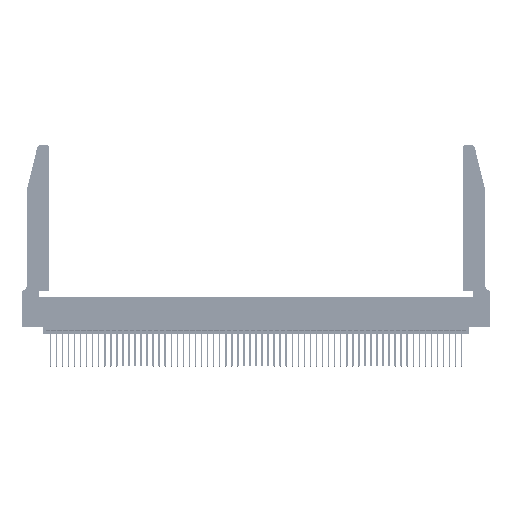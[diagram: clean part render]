
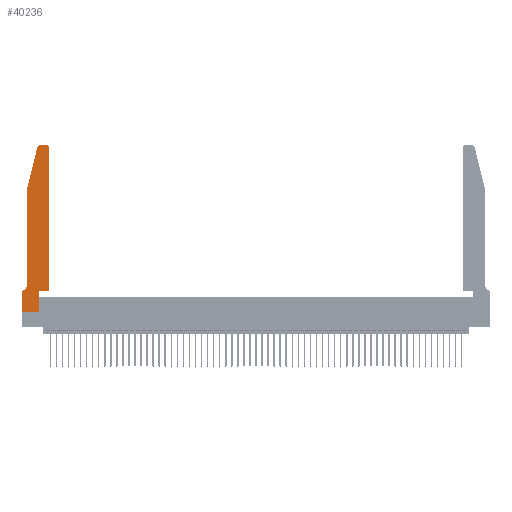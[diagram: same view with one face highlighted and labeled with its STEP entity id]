
A CAD part, top view. The second image highlights one B-rep face of the part: STEP entity #40236.
In plain terms, the highlighted planar face has unit normal (0, 0, 1).
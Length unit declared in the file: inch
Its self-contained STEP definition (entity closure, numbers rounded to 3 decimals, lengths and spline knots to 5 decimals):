
#843 = VERTEX_POINT ( 'NONE', #5994 ) ;
#1290 = VECTOR ( 'NONE', #5709, 39.37008 ) ;
#2330 = CARTESIAN_POINT ( 'NONE',  ( 0.2865, 0.35, 0.37 ) ) ;
#2809 = VECTOR ( 'NONE', #51242, 39.37008 ) ;
#3226 = CARTESIAN_POINT ( 'NONE',  ( 0., 0., 0.37 ) ) ;
#4117 = LINE ( 'NONE', #54791, #48259 ) ;
#4334 = DIRECTION ( 'NONE',  ( 0., 0., 1. ) ) ;
#5709 = DIRECTION ( 'NONE',  ( -1., 0., 0. ) ) ;
#5994 = CARTESIAN_POINT ( 'NONE',  ( 0.0755, 2., 0.37 ) ) ;
#8335 = ORIENTED_EDGE ( 'NONE', *, *, #11516, .T. ) ;
#8473 = ORIENTED_EDGE ( 'NONE', *, *, #53986, .T. ) ;
#9261 = EDGE_CURVE ( 'NONE', #17014, #28813, #13754, .T. ) ;
#11332 = AXIS2_PLACEMENT_3D ( 'NONE', #47181, #21536, #51458 ) ;
#11516 = EDGE_CURVE ( 'NONE', #40117, #47106, #32574, .T. ) ;
#13472 = CARTESIAN_POINT ( 'NONE',  ( 0.2865, 0., 0.37 ) ) ;
#13651 = CARTESIAN_POINT ( 'NONE',  ( 0.4505, 0.35, 0.37 ) ) ;
#13754 = LINE ( 'NONE', #36876, #33897 ) ;
#14243 = DIRECTION ( 'NONE',  ( -0.239, -0.971, 0. ) ) ;
#14474 = VERTEX_POINT ( 'NONE', #30161 ) ;
#14698 = ORIENTED_EDGE ( 'NONE', *, *, #45658, .T. ) ;
#15365 = EDGE_CURVE ( 'NONE', #47703, #40117, #45500, .T. ) ;
#15505 = DIRECTION ( 'NONE',  ( 1., 0., 0. ) ) ;
#15656 = VECTOR ( 'NONE', #32827, 39.37008 ) ;
#15974 = CIRCLE ( 'NONE', #35690, 0.03 ) ;
#16179 = EDGE_CURVE ( 'NONE', #47106, #35549, #30157, .T. ) ;
#16192 = DIRECTION ( 'NONE',  ( 1., 0., 0. ) ) ;
#17014 = VERTEX_POINT ( 'NONE', #2330 ) ;
#17879 = DIRECTION ( 'NONE',  ( 0., 0., 1. ) ) ;
#19423 = VECTOR ( 'NONE', #14243, 39.37008 ) ;
#19909 = VERTEX_POINT ( 'NONE', #49953 ) ;
#20004 = EDGE_CURVE ( 'NONE', #35549, #17014, #53239, .T. ) ;
#20867 = ORIENTED_EDGE ( 'NONE', *, *, #46981, .T. ) ;
#21536 = DIRECTION ( 'NONE',  ( 0., 0., -1. ) ) ;
#21582 = CARTESIAN_POINT ( 'NONE',  ( 0.4505, 2.72, 0.37 ) ) ;
#22791 = CARTESIAN_POINT ( 'NONE',  ( 0., 0., 0.37 ) ) ;
#23832 = CARTESIAN_POINT ( 'NONE',  ( 0., 0.35, 0.37 ) ) ;
#24520 = DIRECTION ( 'NONE',  ( 0., -1., 0. ) ) ;
#24998 = EDGE_CURVE ( 'NONE', #29919, #32193, #4117, .T. ) ;
#25555 = LINE ( 'NONE', #13651, #2809 ) ;
#26405 = CARTESIAN_POINT ( 'NONE',  ( 0., 0., 0.37 ) ) ;
#26889 = CIRCLE ( 'NONE', #54121, 0.03 ) ;
#27423 = ORIENTED_EDGE ( 'NONE', *, *, #48617, .T. ) ;
#27934 = AXIS2_PLACEMENT_3D ( 'NONE', #37550, #28924, #16192 ) ;
#28504 = CARTESIAN_POINT ( 'NONE',  ( 0.0755, 2., 0.37 ) ) ;
#28813 = VERTEX_POINT ( 'NONE', #52680 ) ;
#28924 = DIRECTION ( 'NONE',  ( 0., 0., 1. ) ) ;
#29919 = VERTEX_POINT ( 'NONE', #34887 ) ;
#29979 = CARTESIAN_POINT ( 'NONE',  ( 0.284, 2.72, 0.37 ) ) ;
#30157 = LINE ( 'NONE', #22791, #51509 ) ;
#30161 = CARTESIAN_POINT ( 'NONE',  ( 0.0755, 0.42, 0.37 ) ) ;
#31375 = CARTESIAN_POINT ( 'NONE',  ( 0.0755, 0.35, 0.37 ) ) ;
#32193 = VERTEX_POINT ( 'NONE', #44616 ) ;
#32198 = LINE ( 'NONE', #35623, #19423 ) ;
#32574 = LINE ( 'NONE', #3226, #53936 ) ;
#32729 = ORIENTED_EDGE ( 'NONE', *, *, #15365, .T. ) ;
#32827 = DIRECTION ( 'NONE',  ( 0., -1., 0. ) ) ;
#33463 = ORIENTED_EDGE ( 'NONE', *, *, #24998, .T. ) ;
#33897 = VECTOR ( 'NONE', #15505, 39.37008 ) ;
#34292 = DIRECTION ( 'NONE',  ( 1., 0., 0. ) ) ;
#34887 = CARTESIAN_POINT ( 'NONE',  ( 0.4205, 2.75, 0.37 ) ) ;
#35549 = VERTEX_POINT ( 'NONE', #13472 ) ;
#35592 = FACE_OUTER_BOUND ( 'NONE', #37393, .T. ) ;
#35623 = CARTESIAN_POINT ( 'NONE',  ( 0.0755, 2., 0.37 ) ) ;
#35690 = AXIS2_PLACEMENT_3D ( 'NONE', #43542, #17879, #47810 ) ;
#36846 = VERTEX_POINT ( 'NONE', #21582 ) ;
#36876 = CARTESIAN_POINT ( 'NONE',  ( 0.4505, 0.35, 0.37 ) ) ;
#37393 = EDGE_LOOP ( 'NONE', ( #33463, #8473, #44356, #27423, #20867, #32729, #8335, #38619, #43602, #47743, #38857, #14698 ) ) ;
#37550 = CARTESIAN_POINT ( 'NONE',  ( 0., 0.35, 0.37 ) ) ;
#37844 = DIRECTION ( 'NONE',  ( -1., 0., 0. ) ) ;
#38609 = CIRCLE ( 'NONE', #11332, 0.07 ) ;
#38619 = ORIENTED_EDGE ( 'NONE', *, *, #16179, .T. ) ;
#38857 = ORIENTED_EDGE ( 'NONE', *, *, #53991, .T. ) ;
#40117 = VERTEX_POINT ( 'NONE', #23832 ) ;
#40236 = ADVANCED_FACE ( 'NONE', ( #35592 ), #41843, .T. ) ;
#41843 = PLANE ( 'NONE',  #27934 ) ;
#43266 = VECTOR ( 'NONE', #50525, 39.37008 ) ;
#43542 = CARTESIAN_POINT ( 'NONE',  ( 0.4205, 2.72, 0.37 ) ) ;
#43602 = ORIENTED_EDGE ( 'NONE', *, *, #20004, .T. ) ;
#44356 = ORIENTED_EDGE ( 'NONE', *, *, #44451, .T. ) ;
#44451 = EDGE_CURVE ( 'NONE', #19909, #843, #32198, .T. ) ;
#44616 = CARTESIAN_POINT ( 'NONE',  ( 0.284, 2.75, 0.37 ) ) ;
#45500 = LINE ( 'NONE', #31375, #1290 ) ;
#45658 = EDGE_CURVE ( 'NONE', #36846, #29919, #15974, .T. ) ;
#46268 = CARTESIAN_POINT ( 'NONE',  ( 0.2865, 0.35, 0.37 ) ) ;
#46981 = EDGE_CURVE ( 'NONE', #14474, #47703, #38609, .T. ) ;
#47106 = VERTEX_POINT ( 'NONE', #26405 ) ;
#47181 = CARTESIAN_POINT ( 'NONE',  ( 0.0055, 0.42, 0.37 ) ) ;
#47703 = VERTEX_POINT ( 'NONE', #52160 ) ;
#47743 = ORIENTED_EDGE ( 'NONE', *, *, #9261, .T. ) ;
#47810 = DIRECTION ( 'NONE',  ( 1., 0., 0. ) ) ;
#48259 = VECTOR ( 'NONE', #37844, 39.37008 ) ;
#48423 = DIRECTION ( 'NONE',  ( 1., 0., 0. ) ) ;
#48617 = EDGE_CURVE ( 'NONE', #843, #14474, #51102, .T. ) ;
#49953 = CARTESIAN_POINT ( 'NONE',  ( 0.25487, 2.72718, 0.37 ) ) ;
#50525 = DIRECTION ( 'NONE',  ( 0., 1., 0. ) ) ;
#51102 = LINE ( 'NONE', #28504, #15656 ) ;
#51242 = DIRECTION ( 'NONE',  ( 0., 1., 0. ) ) ;
#51458 = DIRECTION ( 'NONE',  ( -1., 0., 0. ) ) ;
#51509 = VECTOR ( 'NONE', #48423, 39.37008 ) ;
#52160 = CARTESIAN_POINT ( 'NONE',  ( 0.0055, 0.35, 0.37 ) ) ;
#52680 = CARTESIAN_POINT ( 'NONE',  ( 0.4505, 0.35, 0.37 ) ) ;
#53239 = LINE ( 'NONE', #46268, #43266 ) ;
#53936 = VECTOR ( 'NONE', #24520, 39.37008 ) ;
#53986 = EDGE_CURVE ( 'NONE', #32193, #19909, #26889, .T. ) ;
#53991 = EDGE_CURVE ( 'NONE', #28813, #36846, #25555, .T. ) ;
#54121 = AXIS2_PLACEMENT_3D ( 'NONE', #29979, #4334, #34292 ) ;
#54791 = CARTESIAN_POINT ( 'NONE',  ( 0.2605, 2.75, 0.37 ) ) ;
